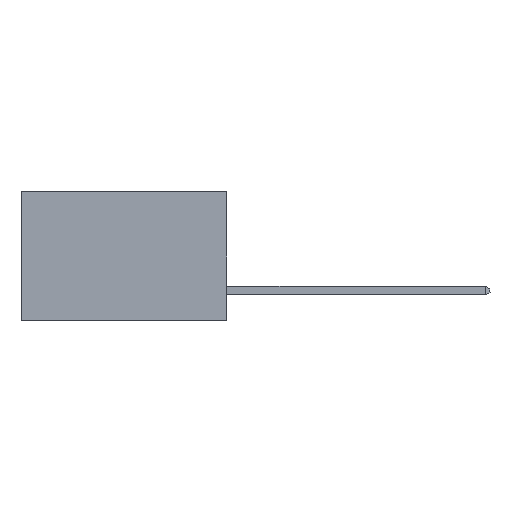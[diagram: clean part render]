
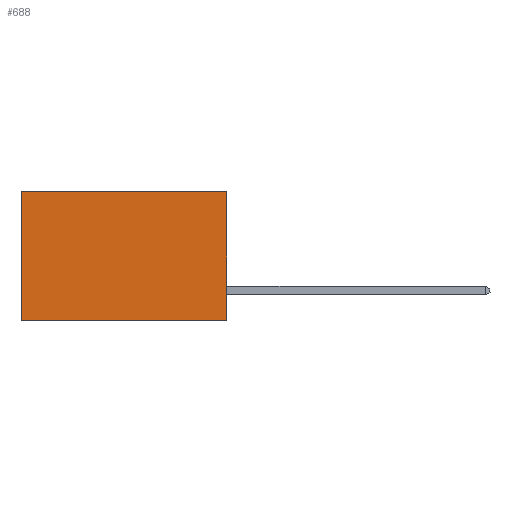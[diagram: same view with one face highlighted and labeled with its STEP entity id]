
A CAD part, left-side view. The second image highlights one B-rep face of the part: STEP entity #688.
In plain terms, the highlighted planar face has unit normal (-1, 0, 0).
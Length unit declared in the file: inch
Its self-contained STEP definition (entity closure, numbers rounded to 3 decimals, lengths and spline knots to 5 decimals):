
#280 = LINE ( 'NONE', #9205, #9240 ) ;
#462 = CARTESIAN_POINT ( 'NONE',  ( 0.277, 0., -0.37 ) ) ;
#493 = LINE ( 'NONE', #5447, #5249 ) ;
#688 = ADVANCED_FACE ( 'NONE', ( #2492 ), #2378, .F. ) ;
#1023 = EDGE_CURVE ( 'NONE', #2677, #6117, #10085, .T. ) ;
#2303 = EDGE_CURVE ( 'NONE', #8418, #6117, #493, .T. ) ;
#2378 = PLANE ( 'NONE',  #9454 ) ;
#2379 = DIRECTION ( 'NONE',  ( 1., 0., 0. ) ) ;
#2478 = CARTESIAN_POINT ( 'NONE',  ( 0.277, 0., -0.37 ) ) ;
#2492 = FACE_OUTER_BOUND ( 'NONE', #3184, .T. ) ;
#2579 = LINE ( 'NONE', #5111, #10787 ) ;
#2677 = VERTEX_POINT ( 'NONE', #462 ) ;
#3184 = EDGE_LOOP ( 'NONE', ( #3959, #4023, #4211, #4316 ) ) ;
#3336 = DIRECTION ( 'NONE',  ( 0., 1., 0. ) ) ;
#3959 = ORIENTED_EDGE ( 'NONE', *, *, #2303, .T. ) ;
#4023 = ORIENTED_EDGE ( 'NONE', *, *, #1023, .F. ) ;
#4211 = ORIENTED_EDGE ( 'NONE', *, *, #4665, .F. ) ;
#4316 = ORIENTED_EDGE ( 'NONE', *, *, #7556, .T. ) ;
#4453 = DIRECTION ( 'NONE',  ( 0., 1., 0. ) ) ;
#4485 = CARTESIAN_POINT ( 'NONE',  ( 0.277, 0., -0.37 ) ) ;
#4665 = EDGE_CURVE ( 'NONE', #9698, #2677, #280, .T. ) ;
#5111 = CARTESIAN_POINT ( 'NONE',  ( 0.277, 0., 0. ) ) ;
#5249 = VECTOR ( 'NONE', #9272, 39.37008 ) ;
#5264 = DIRECTION ( 'NONE',  ( 0., 0., -1. ) ) ;
#5447 = CARTESIAN_POINT ( 'NONE',  ( 0.277, 0.59, -0.37 ) ) ;
#6117 = VERTEX_POINT ( 'NONE', #6653 ) ;
#6433 = CARTESIAN_POINT ( 'NONE',  ( 0.277, 0.59, 0. ) ) ;
#6653 = CARTESIAN_POINT ( 'NONE',  ( 0.277, 0.59, -0.37 ) ) ;
#7556 = EDGE_CURVE ( 'NONE', #9698, #8418, #2579, .T. ) ;
#8167 = VECTOR ( 'NONE', #4453, 39.37008 ) ;
#8418 = VERTEX_POINT ( 'NONE', #6433 ) ;
#8957 = CARTESIAN_POINT ( 'NONE',  ( 0.277, 0., 0. ) ) ;
#9067 = DIRECTION ( 'NONE',  ( 0., 0., -1. ) ) ;
#9205 = CARTESIAN_POINT ( 'NONE',  ( 0.277, 0., -0.37 ) ) ;
#9240 = VECTOR ( 'NONE', #9067, 39.37008 ) ;
#9272 = DIRECTION ( 'NONE',  ( 0., 0., -1. ) ) ;
#9454 = AXIS2_PLACEMENT_3D ( 'NONE', #2478, #2379, #5264 ) ;
#9698 = VERTEX_POINT ( 'NONE', #8957 ) ;
#10085 = LINE ( 'NONE', #4485, #8167 ) ;
#10787 = VECTOR ( 'NONE', #3336, 39.37008 ) ;
